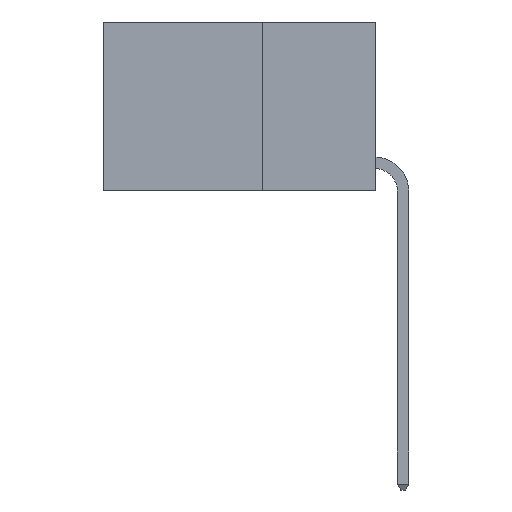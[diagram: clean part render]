
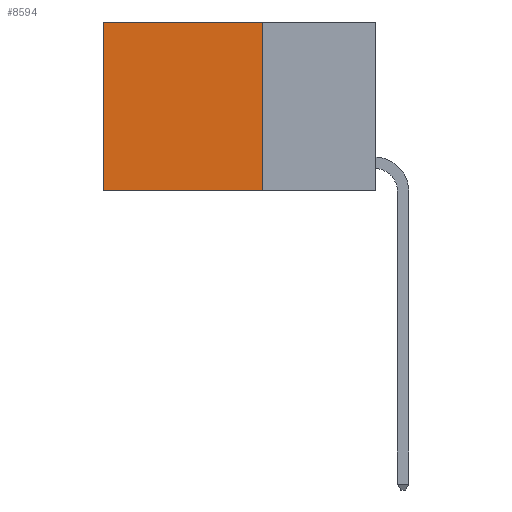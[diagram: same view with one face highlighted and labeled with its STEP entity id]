
A CAD part, left-side view. The second image highlights one B-rep face of the part: STEP entity #8594.
In plain terms, the highlighted planar face has unit normal (-1, 0, 0).
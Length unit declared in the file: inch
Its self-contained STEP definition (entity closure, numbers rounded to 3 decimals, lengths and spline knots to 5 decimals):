
#750 = CARTESIAN_POINT ( 'NONE',  ( 0.2625, 0.25, 0. ) ) ;
#909 = DIRECTION ( 'NONE',  ( 0., 1., 0. ) ) ;
#1180 = FACE_OUTER_BOUND ( 'NONE', #12268, .T. ) ;
#1665 = ORIENTED_EDGE ( 'NONE', *, *, #7035, .T. ) ;
#2027 = VECTOR ( 'NONE', #4297, 39.37008 ) ;
#2259 = CARTESIAN_POINT ( 'NONE',  ( 0.2625, 0.6, 0. ) ) ;
#2561 = VECTOR ( 'NONE', #9769, 39.37008 ) ;
#2986 = LINE ( 'NONE', #15237, #12502 ) ;
#3175 = LINE ( 'NONE', #10228, #2027 ) ;
#3959 = VERTEX_POINT ( 'NONE', #11160 ) ;
#4297 = DIRECTION ( 'NONE',  ( 0., 1., 0. ) ) ;
#4418 = PLANE ( 'NONE',  #6319 ) ;
#4963 = EDGE_CURVE ( 'NONE', #12900, #8144, #2986, .T. ) ;
#5518 = VERTEX_POINT ( 'NONE', #5655 ) ;
#5626 = DIRECTION ( 'NONE',  ( 1., 0., 0. ) ) ;
#5655 = CARTESIAN_POINT ( 'NONE',  ( 0.2625, 0.25, -0.37 ) ) ;
#6319 = AXIS2_PLACEMENT_3D ( 'NONE', #11550, #5626, #13899 ) ;
#6820 = EDGE_CURVE ( 'NONE', #12900, #5518, #13922, .T. ) ;
#7035 = EDGE_CURVE ( 'NONE', #8144, #3959, #14846, .T. ) ;
#8144 = VERTEX_POINT ( 'NONE', #2259 ) ;
#8594 = ADVANCED_FACE ( 'NONE', ( #1180 ), #4418, .F. ) ;
#9164 = EDGE_CURVE ( 'NONE', #5518, #3959, #3175, .T. ) ;
#9575 = CARTESIAN_POINT ( 'NONE',  ( 0.2625, 0.25, 0. ) ) ;
#9769 = DIRECTION ( 'NONE',  ( 0., 0., -1. ) ) ;
#10228 = CARTESIAN_POINT ( 'NONE',  ( 0.2625, 0.25, -0.37 ) ) ;
#10794 = VECTOR ( 'NONE', #11545, 39.37008 ) ;
#11160 = CARTESIAN_POINT ( 'NONE',  ( 0.2625, 0.6, -0.37 ) ) ;
#11545 = DIRECTION ( 'NONE',  ( 0., 0., -1. ) ) ;
#11550 = CARTESIAN_POINT ( 'NONE',  ( 0.2625, 0.25, 0. ) ) ;
#12268 = EDGE_LOOP ( 'NONE', ( #1665, #13433, #13005, #12379 ) ) ;
#12379 = ORIENTED_EDGE ( 'NONE', *, *, #4963, .T. ) ;
#12502 = VECTOR ( 'NONE', #909, 39.37008 ) ;
#12900 = VERTEX_POINT ( 'NONE', #9575 ) ;
#13005 = ORIENTED_EDGE ( 'NONE', *, *, #6820, .F. ) ;
#13283 = CARTESIAN_POINT ( 'NONE',  ( 0.2625, 0.6, 0. ) ) ;
#13433 = ORIENTED_EDGE ( 'NONE', *, *, #9164, .F. ) ;
#13899 = DIRECTION ( 'NONE',  ( 0., 0., -1. ) ) ;
#13922 = LINE ( 'NONE', #750, #10794 ) ;
#14846 = LINE ( 'NONE', #13283, #2561 ) ;
#15237 = CARTESIAN_POINT ( 'NONE',  ( 0.2625, 0.25, 0. ) ) ;
